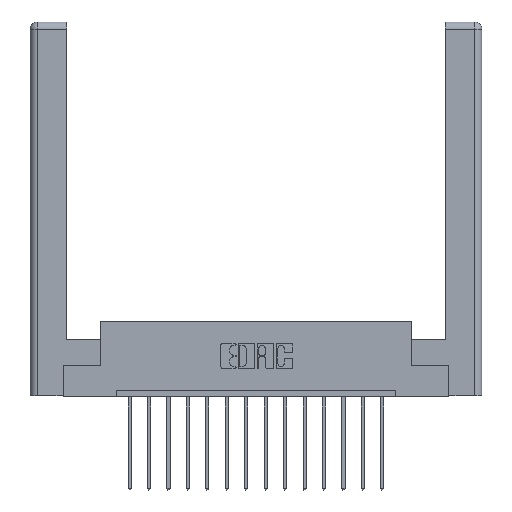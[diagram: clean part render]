
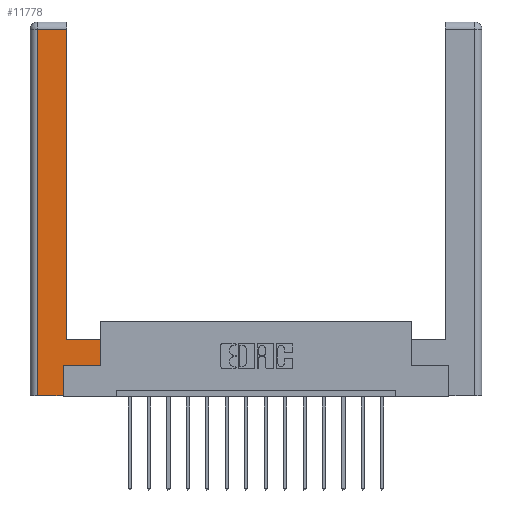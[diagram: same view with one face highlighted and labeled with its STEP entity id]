
A CAD part, top view. The second image highlights one B-rep face of the part: STEP entity #11778.
In plain terms, the highlighted planar face has unit normal (0, 0, 1).
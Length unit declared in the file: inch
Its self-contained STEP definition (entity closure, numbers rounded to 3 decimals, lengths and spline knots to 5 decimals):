
#268 = CARTESIAN_POINT ( 'NONE',  ( 0.0615, 2.94, 0. ) ) ;
#522 = ORIENTED_EDGE ( 'NONE', *, *, #877, .T. ) ;
#608 = ORIENTED_EDGE ( 'NONE', *, *, #862, .T. ) ;
#862 = EDGE_CURVE ( 'NONE', #2723, #4659, #8584, .T. ) ;
#877 = EDGE_CURVE ( 'NONE', #14038, #10873, #11047, .T. ) ;
#918 = CARTESIAN_POINT ( 'NONE',  ( 0.0615, 2.94, 0. ) ) ;
#1089 = DIRECTION ( 'NONE',  ( 0., 1., 0. ) ) ;
#1290 = CARTESIAN_POINT ( 'NONE',  ( 0.295, 3., 0. ) ) ;
#1366 = ORIENTED_EDGE ( 'NONE', *, *, #11338, .T. ) ;
#1423 = DIRECTION ( 'NONE',  ( -1., 0., 0. ) ) ;
#1754 = LINE ( 'NONE', #7521, #3969 ) ;
#2376 = CARTESIAN_POINT ( 'NONE',  ( 0.0615, 0., 0. ) ) ;
#2393 = ORIENTED_EDGE ( 'NONE', *, *, #12830, .T. ) ;
#2512 = DIRECTION ( 'NONE',  ( 0., 1., 0. ) ) ;
#2615 = DIRECTION ( 'NONE',  ( -1., 0., 0. ) ) ;
#2661 = VECTOR ( 'NONE', #2512, 39.37008 ) ;
#2723 = VERTEX_POINT ( 'NONE', #4907 ) ;
#2919 = VECTOR ( 'NONE', #1089, 39.37008 ) ;
#3757 = VECTOR ( 'NONE', #14277, 39.37008 ) ;
#3927 = CARTESIAN_POINT ( 'NONE',  ( 0.0615, 0., 0. ) ) ;
#3969 = VECTOR ( 'NONE', #10170, 39.37008 ) ;
#4051 = VERTEX_POINT ( 'NONE', #268 ) ;
#4306 = EDGE_CURVE ( 'NONE', #4659, #11289, #15136, .T. ) ;
#4329 = ORIENTED_EDGE ( 'NONE', *, *, #4306, .T. ) ;
#4659 = VERTEX_POINT ( 'NONE', #5171 ) ;
#4728 = CARTESIAN_POINT ( 'NONE',  ( 0.565, 0.245, 0. ) ) ;
#4825 = CARTESIAN_POINT ( 'NONE',  ( 0.265, 0.245, 0. ) ) ;
#4907 = CARTESIAN_POINT ( 'NONE',  ( 0.265, 0., 0. ) ) ;
#5171 = CARTESIAN_POINT ( 'NONE',  ( 0.265, 0.245, 0. ) ) ;
#5273 = CARTESIAN_POINT ( 'NONE',  ( 0.565, 0.45, 0. ) ) ;
#6170 = CARTESIAN_POINT ( 'NONE',  ( 0.565, 0.245, 0. ) ) ;
#6269 = PLANE ( 'NONE',  #6689 ) ;
#6542 = CARTESIAN_POINT ( 'NONE',  ( 0., 0., 0. ) ) ;
#6689 = AXIS2_PLACEMENT_3D ( 'NONE', #6542, #9159, #1423 ) ;
#7186 = CARTESIAN_POINT ( 'NONE',  ( 0.295, 2.94, 0. ) ) ;
#7273 = DIRECTION ( 'NONE',  ( 1., 0., 0. ) ) ;
#7521 = CARTESIAN_POINT ( 'NONE',  ( 0.265, 0., 0. ) ) ;
#7829 = LINE ( 'NONE', #1290, #15118 ) ;
#8020 = EDGE_LOOP ( 'NONE', ( #2393, #1366, #11276, #14953, #608, #4329, #11640, #522 ) ) ;
#8075 = LINE ( 'NONE', #918, #14144 ) ;
#8480 = FACE_OUTER_BOUND ( 'NONE', #8020, .T. ) ;
#8556 = EDGE_CURVE ( 'NONE', #9785, #2723, #1754, .T. ) ;
#8584 = LINE ( 'NONE', #4825, #2919 ) ;
#8729 = DIRECTION ( 'NONE',  ( -1., 0., 0. ) ) ;
#9159 = DIRECTION ( 'NONE',  ( 0., 0., -1. ) ) ;
#9742 = LINE ( 'NONE', #15502, #2661 ) ;
#9785 = VERTEX_POINT ( 'NONE', #2376 ) ;
#9826 = LINE ( 'NONE', #3927, #3757 ) ;
#10074 = VECTOR ( 'NONE', #7273, 39.37008 ) ;
#10170 = DIRECTION ( 'NONE',  ( 1., 0., 0. ) ) ;
#10873 = VERTEX_POINT ( 'NONE', #14455 ) ;
#11047 = LINE ( 'NONE', #12755, #12850 ) ;
#11276 = ORIENTED_EDGE ( 'NONE', *, *, #13487, .T. ) ;
#11289 = VERTEX_POINT ( 'NONE', #6170 ) ;
#11338 = EDGE_CURVE ( 'NONE', #16286, #4051, #8075, .T. ) ;
#11640 = ORIENTED_EDGE ( 'NONE', *, *, #15932, .T. ) ;
#11778 = ADVANCED_FACE ( 'NONE', ( #8480 ), #6269, .F. ) ;
#12755 = CARTESIAN_POINT ( 'NONE',  ( 0.295, 0.45, 0. ) ) ;
#12830 = EDGE_CURVE ( 'NONE', #10873, #16286, #7829, .T. ) ;
#12850 = VECTOR ( 'NONE', #8729, 39.37008 ) ;
#13487 = EDGE_CURVE ( 'NONE', #4051, #9785, #9826, .T. ) ;
#14038 = VERTEX_POINT ( 'NONE', #5273 ) ;
#14144 = VECTOR ( 'NONE', #2615, 39.37008 ) ;
#14277 = DIRECTION ( 'NONE',  ( 0., -1., 0. ) ) ;
#14455 = CARTESIAN_POINT ( 'NONE',  ( 0.295, 0.45, 0. ) ) ;
#14953 = ORIENTED_EDGE ( 'NONE', *, *, #8556, .T. ) ;
#15118 = VECTOR ( 'NONE', #16672, 39.37008 ) ;
#15136 = LINE ( 'NONE', #4728, #10074 ) ;
#15502 = CARTESIAN_POINT ( 'NONE',  ( 0.565, 0.45, 0. ) ) ;
#15932 = EDGE_CURVE ( 'NONE', #11289, #14038, #9742, .T. ) ;
#16286 = VERTEX_POINT ( 'NONE', #7186 ) ;
#16672 = DIRECTION ( 'NONE',  ( 0., 1., 0. ) ) ;
